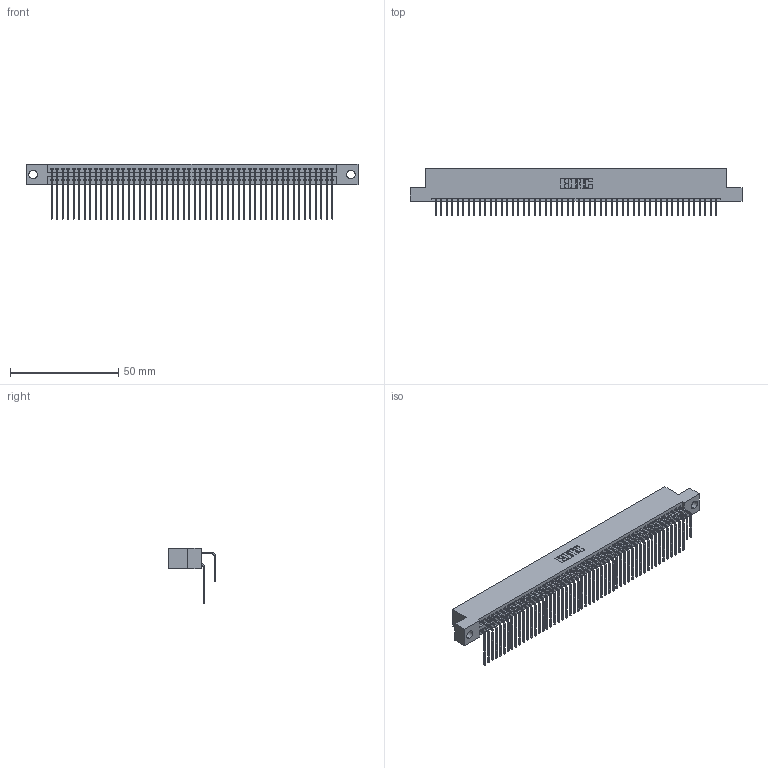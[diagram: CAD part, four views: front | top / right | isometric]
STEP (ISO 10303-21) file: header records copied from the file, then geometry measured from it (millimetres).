
FILE_DESCRIPTION (( 'STEP AP203' ), '1' );
FILE_NAME ('395-104-558-204.STEP', '2021-06-17T16:15:49', ( '' ), ( '' ), 'SwSTEP 2.0', 'SolidWorks 2020', '' );
FILE_SCHEMA (( 'CONFIG_CONTROL_DESIGN' ));
Length unit declared in the file: inch
Products named in the file (4): 345-292-001_558 Tail - 2; 345-292-001_558 559 Tail - 1; 345 Part_Flush Mounting Lugs - 0.156 Dia-TI; 395-104-558-204
Assembly tree (105 placements, depth 2):
  395-104-558-204
    345 Part_Flush Mounting Lugs - 0.156 Dia-TI
    345-292-001_558 559 Tail - 1  x52
    345-292-001_558 Tail - 2  x52
Bounding box: 153.29 x 21.83 x 25.53 mm (x, y, z)
Volume: 15477.5 mm3; surface area: 25744.7 mm2
Topology: 105 solids, 105 shells, 5548 faces, 16497 edges, 10858 vertices
Faces by surface type: plane 3734, cylinder 1814
Entity records: 41525 total; most frequent: CARTESIAN_POINT 7001, ORIENTED_EDGE 6882, DIRECTION 6133, EDGE_CURVE 3441, VECTOR 3061, LINE 3061, VERTEX_POINT 2290, AXIS2_PLACEMENT_3D 1536
